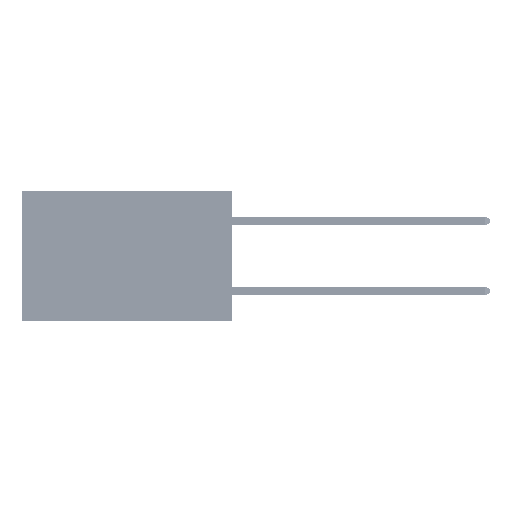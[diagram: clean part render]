
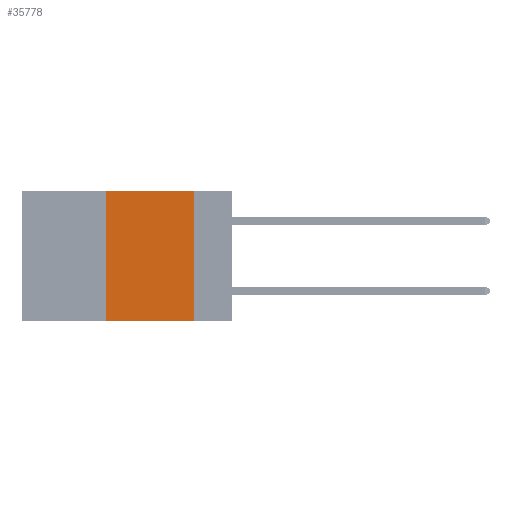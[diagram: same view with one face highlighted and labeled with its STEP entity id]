
A CAD part, left-side view. The second image highlights one B-rep face of the part: STEP entity #35778.
In plain terms, the highlighted planar face has unit normal (-1, 0, 0).
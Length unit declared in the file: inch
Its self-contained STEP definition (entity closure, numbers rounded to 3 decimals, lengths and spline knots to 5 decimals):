
#440 = VERTEX_POINT ( 'NONE', #25729 ) ;
#2353 = VECTOR ( 'NONE', #24654, 39.37008 ) ;
#2515 = VECTOR ( 'NONE', #10259, 39.37008 ) ;
#3000 = VECTOR ( 'NONE', #36496, 39.37008 ) ;
#4013 = CARTESIAN_POINT ( 'NONE',  ( 0., 0.6, 0. ) ) ;
#4098 = PLANE ( 'NONE',  #40186 ) ;
#4913 = EDGE_CURVE ( 'NONE', #17221, #440, #7719, .T. ) ;
#5236 = EDGE_LOOP ( 'NONE', ( #47025, #40247, #39201, #12139 ) ) ;
#7719 = LINE ( 'NONE', #24990, #3000 ) ;
#8236 = EDGE_CURVE ( 'NONE', #27030, #17221, #17956, .T. ) ;
#10259 = DIRECTION ( 'NONE',  ( 0., 0., 1. ) ) ;
#11392 = DIRECTION ( 'NONE',  ( 0., -1., 0. ) ) ;
#12139 = ORIENTED_EDGE ( 'NONE', *, *, #30378, .T. ) ;
#13663 = CARTESIAN_POINT ( 'NONE',  ( 0., 0.36, -0.37 ) ) ;
#15790 = VERTEX_POINT ( 'NONE', #13663 ) ;
#17221 = VERTEX_POINT ( 'NONE', #22379 ) ;
#17459 = CARTESIAN_POINT ( 'NONE',  ( 0., 0.36, 0. ) ) ;
#17867 = CARTESIAN_POINT ( 'NONE',  ( 0., 0.36, 0. ) ) ;
#17956 = LINE ( 'NONE', #4013, #45132 ) ;
#19653 = DIRECTION ( 'NONE',  ( 1., 0., 0. ) ) ;
#21314 = CARTESIAN_POINT ( 'NONE',  ( 0., 0.6, -0.37 ) ) ;
#22379 = CARTESIAN_POINT ( 'NONE',  ( 0., 0.11, 0. ) ) ;
#24654 = DIRECTION ( 'NONE',  ( 0., -1., 0. ) ) ;
#24990 = CARTESIAN_POINT ( 'NONE',  ( 0., 0.11, 0. ) ) ;
#25729 = CARTESIAN_POINT ( 'NONE',  ( 0., 0.11, -0.37 ) ) ;
#27030 = VERTEX_POINT ( 'NONE', #17867 ) ;
#30371 = CARTESIAN_POINT ( 'NONE',  ( 0., 0.6, 0. ) ) ;
#30378 = EDGE_CURVE ( 'NONE', #15790, #440, #32326, .T. ) ;
#32326 = LINE ( 'NONE', #21314, #2353 ) ;
#35778 = ADVANCED_FACE ( 'NONE', ( #44824 ), #4098, .F. ) ;
#36496 = DIRECTION ( 'NONE',  ( 0., 0., -1. ) ) ;
#38613 = DIRECTION ( 'NONE',  ( 0., 0., -1. ) ) ;
#39201 = ORIENTED_EDGE ( 'NONE', *, *, #41339, .F. ) ;
#40186 = AXIS2_PLACEMENT_3D ( 'NONE', #30371, #19653, #38613 ) ;
#40247 = ORIENTED_EDGE ( 'NONE', *, *, #8236, .F. ) ;
#41313 = LINE ( 'NONE', #17459, #2515 ) ;
#41339 = EDGE_CURVE ( 'NONE', #15790, #27030, #41313, .T. ) ;
#44824 = FACE_OUTER_BOUND ( 'NONE', #5236, .T. ) ;
#45132 = VECTOR ( 'NONE', #11392, 39.37008 ) ;
#47025 = ORIENTED_EDGE ( 'NONE', *, *, #4913, .F. ) ;
